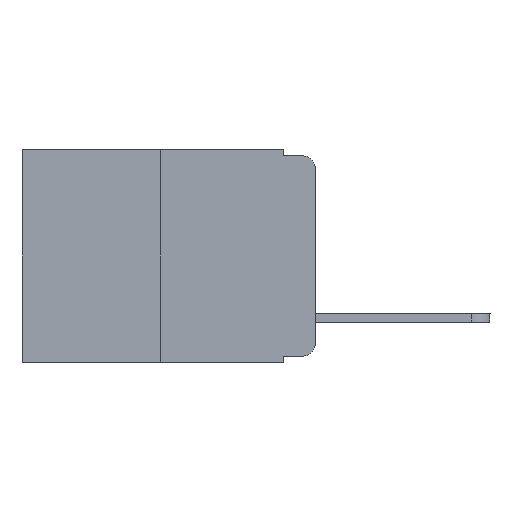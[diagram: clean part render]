
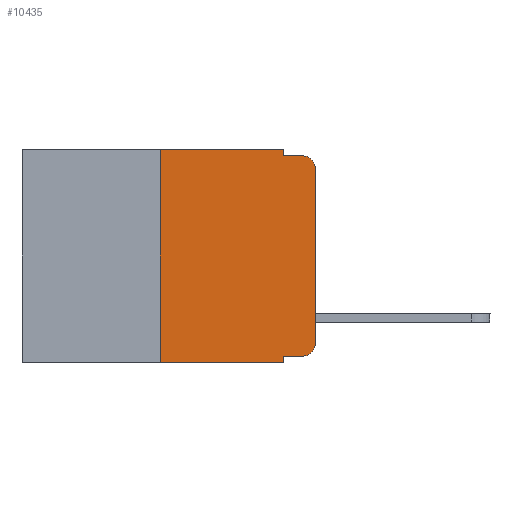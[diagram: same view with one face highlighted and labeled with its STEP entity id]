
A CAD part, left-side view. The second image highlights one B-rep face of the part: STEP entity #10435.
In plain terms, the highlighted planar face has unit normal (-1, 0, 0).
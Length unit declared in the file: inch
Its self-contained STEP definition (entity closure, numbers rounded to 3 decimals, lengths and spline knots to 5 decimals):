
#24 = CARTESIAN_POINT ( 'NONE',  ( 0., 0., -0.03 ) ) ;
#124 = VERTEX_POINT ( 'NONE', #10334 ) ;
#392 = VERTEX_POINT ( 'NONE', #10499 ) ;
#395 = CARTESIAN_POINT ( 'NONE',  ( 0., 0.02, -0.333 ) ) ;
#451 = ORIENTED_EDGE ( 'NONE', *, *, #2383, .T. ) ;
#482 = VERTEX_POINT ( 'NONE', #7465 ) ;
#538 = CARTESIAN_POINT ( 'NONE',  ( 0., 0.473, 0. ) ) ;
#660 = LINE ( 'NONE', #6384, #5566 ) ;
#770 = EDGE_CURVE ( 'NONE', #2128, #124, #2150, .T. ) ;
#1171 = LINE ( 'NONE', #8697, #2452 ) ;
#1226 = CARTESIAN_POINT ( 'NONE',  ( 0., 0., 0. ) ) ;
#1250 = ORIENTED_EDGE ( 'NONE', *, *, #7808, .T. ) ;
#1284 = DIRECTION ( 'NONE',  ( 0., 0., -1. ) ) ;
#1414 = CARTESIAN_POINT ( 'NONE',  ( 0., 0.051, -0.333 ) ) ;
#1425 = VECTOR ( 'NONE', #8241, 39.37008 ) ;
#1663 = CARTESIAN_POINT ( 'NONE',  ( 0., 0.473, -0.343 ) ) ;
#1723 = EDGE_CURVE ( 'NONE', #7679, #392, #1171, .T. ) ;
#1842 = VERTEX_POINT ( 'NONE', #3984 ) ;
#1858 = CARTESIAN_POINT ( 'NONE',  ( 0., 0.02, -0.03 ) ) ;
#2128 = VERTEX_POINT ( 'NONE', #3489 ) ;
#2150 = LINE ( 'NONE', #9995, #6539 ) ;
#2383 = EDGE_CURVE ( 'NONE', #7679, #482, #9841, .T. ) ;
#2426 = DIRECTION ( 'NONE',  ( 0., -1., 0. ) ) ;
#2452 = VECTOR ( 'NONE', #9681, 39.37008 ) ;
#2563 = DIRECTION ( 'NONE',  ( 0., -1., 0. ) ) ;
#2801 = EDGE_LOOP ( 'NONE', ( #1250, #6177, #4054, #6417, #7755, #10049, #451, #3272, #3547, #8079 ) ) ;
#3028 = VECTOR ( 'NONE', #9679, 39.37008 ) ;
#3272 = ORIENTED_EDGE ( 'NONE', *, *, #5852, .F. ) ;
#3398 = VECTOR ( 'NONE', #6714, 39.37008 ) ;
#3489 = CARTESIAN_POINT ( 'NONE',  ( 0., 0.051, -0.01 ) ) ;
#3547 = ORIENTED_EDGE ( 'NONE', *, *, #7482, .T. ) ;
#3566 = VECTOR ( 'NONE', #2563, 39.37008 ) ;
#3931 = PLANE ( 'NONE',  #10238 ) ;
#3984 = CARTESIAN_POINT ( 'NONE',  ( 0., 0.051, 0. ) ) ;
#4054 = ORIENTED_EDGE ( 'NONE', *, *, #770, .F. ) ;
#4472 = CARTESIAN_POINT ( 'NONE',  ( 0., 0.25, -0.343 ) ) ;
#4487 = CARTESIAN_POINT ( 'NONE',  ( 0., 0., -0.313 ) ) ;
#4765 = DIRECTION ( 'NONE',  ( -1., 0., 0. ) ) ;
#4780 = CIRCLE ( 'NONE', #8926, 0.02 ) ;
#4863 = LINE ( 'NONE', #10660, #3566 ) ;
#5385 = LINE ( 'NONE', #1226, #3028 ) ;
#5407 = VERTEX_POINT ( 'NONE', #4487 ) ;
#5566 = VECTOR ( 'NONE', #7208, 39.37008 ) ;
#5718 = DIRECTION ( 'NONE',  ( 0., -1., 0. ) ) ;
#5852 = EDGE_CURVE ( 'NONE', #6062, #482, #9872, .T. ) ;
#5989 = VECTOR ( 'NONE', #2426, 39.37008 ) ;
#6056 = DIRECTION ( 'NONE',  ( 0., 0., -1. ) ) ;
#6062 = VERTEX_POINT ( 'NONE', #1414 ) ;
#6151 = AXIS2_PLACEMENT_3D ( 'NONE', #7253, #4765, #8928 ) ;
#6177 = ORIENTED_EDGE ( 'NONE', *, *, #7235, .T. ) ;
#6384 = CARTESIAN_POINT ( 'NONE',  ( 0., 0.051, 0. ) ) ;
#6417 = ORIENTED_EDGE ( 'NONE', *, *, #10205, .F. ) ;
#6539 = VECTOR ( 'NONE', #5718, 39.37008 ) ;
#6714 = DIRECTION ( 'NONE',  ( 0., -1., 0. ) ) ;
#7208 = DIRECTION ( 'NONE',  ( 0., 0., -1. ) ) ;
#7235 = EDGE_CURVE ( 'NONE', #9106, #124, #4780, .T. ) ;
#7253 = CARTESIAN_POINT ( 'NONE',  ( 0., 0.02, -0.313 ) ) ;
#7352 = EDGE_CURVE ( 'NONE', #8554, #5407, #7708, .T. ) ;
#7465 = CARTESIAN_POINT ( 'NONE',  ( 0., 0.051, -0.343 ) ) ;
#7482 = EDGE_CURVE ( 'NONE', #6062, #8554, #4863, .T. ) ;
#7497 = EDGE_CURVE ( 'NONE', #392, #1842, #9141, .T. ) ;
#7519 = CARTESIAN_POINT ( 'NONE',  ( 0., 0.473, 0. ) ) ;
#7628 = DIRECTION ( 'NONE',  ( -1., 0., 0. ) ) ;
#7679 = VERTEX_POINT ( 'NONE', #4472 ) ;
#7708 = CIRCLE ( 'NONE', #6151, 0.02 ) ;
#7755 = ORIENTED_EDGE ( 'NONE', *, *, #7497, .F. ) ;
#7808 = EDGE_CURVE ( 'NONE', #5407, #9106, #5385, .T. ) ;
#7814 = FACE_OUTER_BOUND ( 'NONE', #2801, .T. ) ;
#8079 = ORIENTED_EDGE ( 'NONE', *, *, #7352, .T. ) ;
#8241 = DIRECTION ( 'NONE',  ( 0., 0., -1. ) ) ;
#8554 = VERTEX_POINT ( 'NONE', #395 ) ;
#8697 = CARTESIAN_POINT ( 'NONE',  ( 0., 0.25, 0. ) ) ;
#8926 = AXIS2_PLACEMENT_3D ( 'NONE', #1858, #7628, #6056 ) ;
#8928 = DIRECTION ( 'NONE',  ( 0., 0., -1. ) ) ;
#9045 = CARTESIAN_POINT ( 'NONE',  ( 0., 0.051, 0. ) ) ;
#9106 = VERTEX_POINT ( 'NONE', #24 ) ;
#9141 = LINE ( 'NONE', #7519, #3398 ) ;
#9679 = DIRECTION ( 'NONE',  ( 0., 0., 1. ) ) ;
#9681 = DIRECTION ( 'NONE',  ( 0., 0., 1. ) ) ;
#9841 = LINE ( 'NONE', #1663, #5989 ) ;
#9872 = LINE ( 'NONE', #9045, #1425 ) ;
#9995 = CARTESIAN_POINT ( 'NONE',  ( 0., 0.051, -0.01 ) ) ;
#10049 = ORIENTED_EDGE ( 'NONE', *, *, #1723, .F. ) ;
#10205 = EDGE_CURVE ( 'NONE', #1842, #2128, #660, .T. ) ;
#10238 = AXIS2_PLACEMENT_3D ( 'NONE', #538, #10535, #1284 ) ;
#10334 = CARTESIAN_POINT ( 'NONE',  ( 0., 0.02, -0.01 ) ) ;
#10435 = ADVANCED_FACE ( 'NONE', ( #7814 ), #3931, .F. ) ;
#10499 = CARTESIAN_POINT ( 'NONE',  ( 0., 0.25, 0. ) ) ;
#10535 = DIRECTION ( 'NONE',  ( 1., 0., 0. ) ) ;
#10660 = CARTESIAN_POINT ( 'NONE',  ( 0., 0.051, -0.333 ) ) ;
